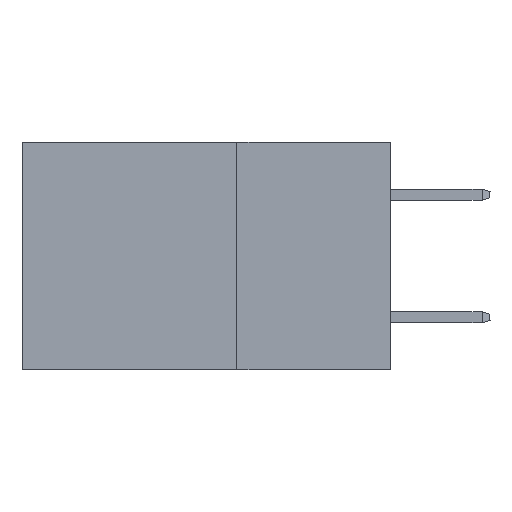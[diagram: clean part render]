
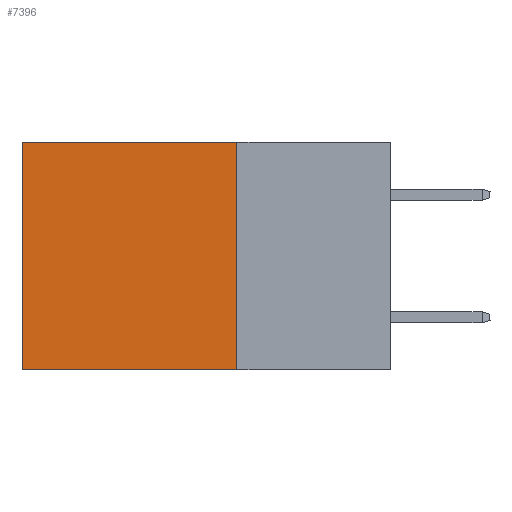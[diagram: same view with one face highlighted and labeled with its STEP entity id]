
A CAD part, left-side view. The second image highlights one B-rep face of the part: STEP entity #7396.
In plain terms, the highlighted planar face has unit normal (-1, 0, 0).
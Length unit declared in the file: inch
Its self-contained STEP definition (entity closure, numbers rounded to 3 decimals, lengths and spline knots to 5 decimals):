
#1845 = DIRECTION ( 'NONE',  ( 0., 0., -1. ) ) ;
#7396 = ADVANCED_FACE ( 'NONE', ( #29766 ), #11153, .F. ) ;
#8581 = CARTESIAN_POINT ( 'NONE',  ( 0.2875, 0.25, -0.37 ) ) ;
#9259 = CARTESIAN_POINT ( 'NONE',  ( 0.2875, 0.25, 0. ) ) ;
#9394 = ORIENTED_EDGE ( 'NONE', *, *, #35161, .T. ) ;
#9423 = EDGE_CURVE ( 'NONE', #16204, #10574, #39033, .T. ) ;
#10574 = VERTEX_POINT ( 'NONE', #19726 ) ;
#10662 = ORIENTED_EDGE ( 'NONE', *, *, #23524, .T. ) ;
#10990 = CARTESIAN_POINT ( 'NONE',  ( 0.2875, 0.25, 0. ) ) ;
#11153 = PLANE ( 'NONE',  #35392 ) ;
#13712 = VECTOR ( 'NONE', #18805, 39.37008 ) ;
#14704 = VECTOR ( 'NONE', #20071, 39.37008 ) ;
#15213 = VECTOR ( 'NONE', #29236, 39.37008 ) ;
#16204 = VERTEX_POINT ( 'NONE', #9259 ) ;
#17245 = EDGE_CURVE ( 'NONE', #10574, #31794, #31410, .T. ) ;
#18805 = DIRECTION ( 'NONE',  ( 0., 0., -1. ) ) ;
#19726 = CARTESIAN_POINT ( 'NONE',  ( 0.2875, 0.25, -0.37 ) ) ;
#20071 = DIRECTION ( 'NONE',  ( 0., 1., 0. ) ) ;
#20129 = VERTEX_POINT ( 'NONE', #27888 ) ;
#20950 = LINE ( 'NONE', #32246, #15213 ) ;
#22819 = LINE ( 'NONE', #10990, #14704 ) ;
#23349 = VECTOR ( 'NONE', #39063, 39.37008 ) ;
#23524 = EDGE_CURVE ( 'NONE', #16204, #20129, #22819, .T. ) ;
#26460 = DIRECTION ( 'NONE',  ( 1., 0., 0. ) ) ;
#27888 = CARTESIAN_POINT ( 'NONE',  ( 0.2875, 0.6, 0. ) ) ;
#29236 = DIRECTION ( 'NONE',  ( 0., 0., -1. ) ) ;
#29766 = FACE_OUTER_BOUND ( 'NONE', #37267, .T. ) ;
#30027 = ORIENTED_EDGE ( 'NONE', *, *, #9423, .F. ) ;
#30775 = CARTESIAN_POINT ( 'NONE',  ( 0.2875, 0.6, -0.37 ) ) ;
#31410 = LINE ( 'NONE', #8581, #23349 ) ;
#31794 = VERTEX_POINT ( 'NONE', #30775 ) ;
#32246 = CARTESIAN_POINT ( 'NONE',  ( 0.2875, 0.6, 0. ) ) ;
#32415 = CARTESIAN_POINT ( 'NONE',  ( 0.2875, 0.25, 0. ) ) ;
#34407 = ORIENTED_EDGE ( 'NONE', *, *, #17245, .F. ) ;
#35161 = EDGE_CURVE ( 'NONE', #20129, #31794, #20950, .T. ) ;
#35392 = AXIS2_PLACEMENT_3D ( 'NONE', #32415, #26460, #1845 ) ;
#37267 = EDGE_LOOP ( 'NONE', ( #9394, #34407, #30027, #10662 ) ) ;
#39033 = LINE ( 'NONE', #39255, #13712 ) ;
#39063 = DIRECTION ( 'NONE',  ( 0., 1., 0. ) ) ;
#39255 = CARTESIAN_POINT ( 'NONE',  ( 0.2875, 0.25, 0. ) ) ;
